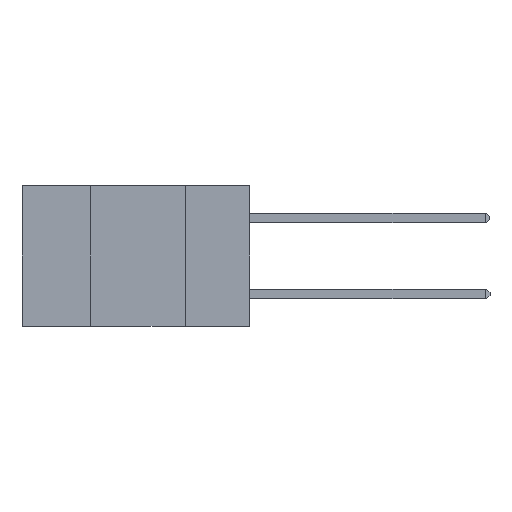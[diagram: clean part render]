
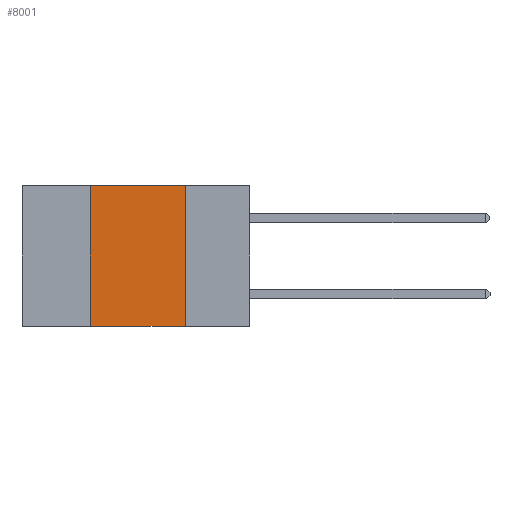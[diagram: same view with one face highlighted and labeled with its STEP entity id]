
A CAD part, left-side view. The second image highlights one B-rep face of the part: STEP entity #8001.
In plain terms, the highlighted planar face has unit normal (-1, 0, 0).
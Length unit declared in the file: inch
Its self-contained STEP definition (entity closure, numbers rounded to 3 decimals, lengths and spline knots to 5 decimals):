
#805 = VERTEX_POINT ( 'NONE', #2639 ) ;
#833 = EDGE_CURVE ( 'NONE', #9669, #8238, #5801, .T. ) ;
#2284 = DIRECTION ( 'NONE',  ( 0., -1., 0. ) ) ;
#2457 = CARTESIAN_POINT ( 'NONE',  ( 0., 0.42, 0. ) ) ;
#2475 = LINE ( 'NONE', #2457, #10152 ) ;
#2639 = CARTESIAN_POINT ( 'NONE',  ( 0., 0.17, 0. ) ) ;
#2998 = PLANE ( 'NONE',  #11275 ) ;
#3450 = DIRECTION ( 'NONE',  ( 0., 0., 1. ) ) ;
#4010 = DIRECTION ( 'NONE',  ( 0., 0., -1. ) ) ;
#4389 = CARTESIAN_POINT ( 'NONE',  ( 0., 0.17, -0.37 ) ) ;
#4437 = VERTEX_POINT ( 'NONE', #11913 ) ;
#4662 = DIRECTION ( 'NONE',  ( 0., -1., 0. ) ) ;
#5063 = EDGE_LOOP ( 'NONE', ( #10952, #9417, #12615, #11270 ) ) ;
#5801 = LINE ( 'NONE', #6340, #8142 ) ;
#5988 = CARTESIAN_POINT ( 'NONE',  ( 0., 0.6, 0. ) ) ;
#6340 = CARTESIAN_POINT ( 'NONE',  ( 0., 0.6, -0.37 ) ) ;
#6815 = VECTOR ( 'NONE', #4662, 39.37008 ) ;
#7504 = CARTESIAN_POINT ( 'NONE',  ( 0., 0.42, -0.37 ) ) ;
#8001 = ADVANCED_FACE ( 'NONE', ( #8602 ), #2998, .F. ) ;
#8142 = VECTOR ( 'NONE', #2284, 39.37008 ) ;
#8238 = VERTEX_POINT ( 'NONE', #4389 ) ;
#8283 = EDGE_CURVE ( 'NONE', #9669, #4437, #2475, .T. ) ;
#8602 = FACE_OUTER_BOUND ( 'NONE', #5063, .T. ) ;
#8702 = LINE ( 'NONE', #9549, #9011 ) ;
#9011 = VECTOR ( 'NONE', #10525, 39.37008 ) ;
#9417 = ORIENTED_EDGE ( 'NONE', *, *, #12632, .F. ) ;
#9549 = CARTESIAN_POINT ( 'NONE',  ( 0., 0.17, 0. ) ) ;
#9669 = VERTEX_POINT ( 'NONE', #7504 ) ;
#9995 = DIRECTION ( 'NONE',  ( 1., 0., 0. ) ) ;
#10023 = EDGE_CURVE ( 'NONE', #805, #8238, #8702, .T. ) ;
#10152 = VECTOR ( 'NONE', #3450, 39.37008 ) ;
#10525 = DIRECTION ( 'NONE',  ( 0., 0., -1. ) ) ;
#10952 = ORIENTED_EDGE ( 'NONE', *, *, #10023, .F. ) ;
#11270 = ORIENTED_EDGE ( 'NONE', *, *, #833, .T. ) ;
#11275 = AXIS2_PLACEMENT_3D ( 'NONE', #5988, #9995, #4010 ) ;
#11913 = CARTESIAN_POINT ( 'NONE',  ( 0., 0.42, 0. ) ) ;
#12370 = LINE ( 'NONE', #12593, #6815 ) ;
#12593 = CARTESIAN_POINT ( 'NONE',  ( 0., 0.6, 0. ) ) ;
#12615 = ORIENTED_EDGE ( 'NONE', *, *, #8283, .F. ) ;
#12632 = EDGE_CURVE ( 'NONE', #4437, #805, #12370, .T. ) ;
